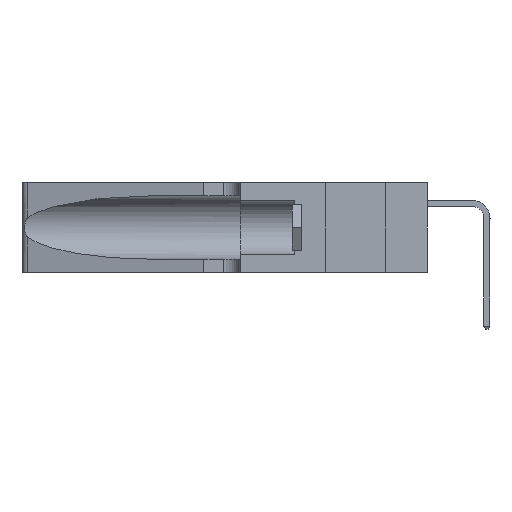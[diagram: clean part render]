
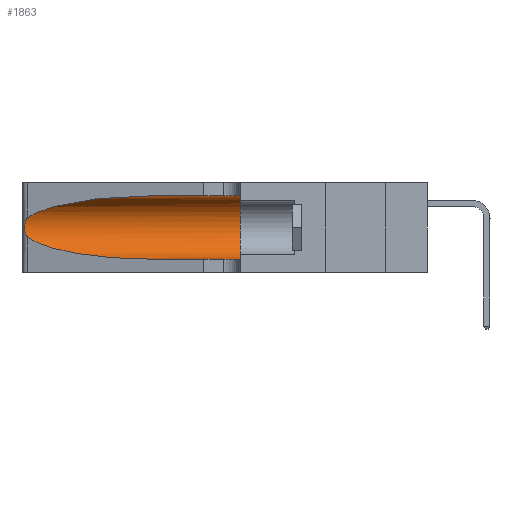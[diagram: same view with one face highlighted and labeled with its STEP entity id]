
A CAD part, left-side view. The second image highlights one B-rep face of the part: STEP entity #1863.
In plain terms, the highlighted cylindrical face has radius 3.308 mm (diameter 6.617 mm), a partial arc.
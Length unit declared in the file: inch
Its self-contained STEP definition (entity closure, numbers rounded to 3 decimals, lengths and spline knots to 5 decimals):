
#24 = DIRECTION ( 'NONE',  ( 0., 0., 1. ) ) ;
#83 = CARTESIAN_POINT ( 'NONE',  ( 0.1305, 0.35, 0.185 ) ) ;
#750 = DIRECTION ( 'NONE',  ( 0., -1., 0. ) ) ;
#790 = EDGE_CURVE ( 'NONE', #14074, #18296, #7745, .T. ) ;
#1110 = ORIENTED_EDGE ( 'NONE', *, *, #6047, .T. ) ;
#1334 = CARTESIAN_POINT ( 'NONE',  ( 0.25854, 1.2359, 0.20912 ) ) ;
#1863 = ADVANCED_FACE ( 'NONE', ( #5632 ), #17298, .F. ) ;
#2097 = LINE ( 'NONE', #19069, #5708 ) ;
#2897 = CARTESIAN_POINT ( 'NONE',  ( 0.26075, 1.23896, 0.19203 ) ) ;
#3001 = VECTOR ( 'NONE', #19380, 39.37008 ) ;
#3007 = CARTESIAN_POINT ( 'NONE',  ( 0.18966, 0.96281, 0.05475 ) ) ;
#3076 = B_SPLINE_CURVE_WITH_KNOTS ( 'NONE', 3,
 ( #5937, #13520, #19613, #10523, #1334, #12057, #2897, #13582, #4463, #15131, #6002, #16643, #7543, #18157 ),
 .UNSPECIFIED., .F., .F.,
 ( 4, 2, 2, 2, 2, 2, 4 ),
 ( 0., 0.00027, 0.00053, 0.00107, 0.0016, 0.00187, 0.00214 ),
 .UNSPECIFIED. ) ;
#3097 = VERTEX_POINT ( 'NONE', #10266 ) ;
#4463 = CARTESIAN_POINT ( 'NONE',  ( 0.26017, 1.23833, 0.17102 ) ) ;
#4508 = CARTESIAN_POINT ( 'NONE',  ( 0.25487, 1.22718, 0.14631 ) ) ;
#4941 = DIRECTION ( 'NONE',  ( 0., 1., 0. ) ) ;
#4996 = CARTESIAN_POINT ( 'NONE',  ( 0.18966, 0.96281, 0.31525 ) ) ;
#5586 = DIRECTION ( 'NONE',  ( 0., -1., 0. ) ) ;
#5632 = FACE_OUTER_BOUND ( 'NONE', #19132, .T. ) ;
#5708 = VECTOR ( 'NONE', #750, 39.37008 ) ;
#5758 = CARTESIAN_POINT ( 'NONE',  ( 0.1305, 1.61858, 0.31525 ) ) ;
#5937 = CARTESIAN_POINT ( 'NONE',  ( 0.25487, 1.22718, 0.22369 ) ) ;
#6002 = CARTESIAN_POINT ( 'NONE',  ( 0.25789, 1.23486, 0.15765 ) ) ;
#6047 = EDGE_CURVE ( 'NONE', #15755, #3097, #17273, .T. ) ;
#7324 = EDGE_CURVE ( 'NONE', #8057, #14074, #15196, .T. ) ;
#7543 = CARTESIAN_POINT ( 'NONE',  ( 0.25555, 1.22993, 0.14849 ) ) ;
#7589 = CARTESIAN_POINT ( 'NONE',  ( 0.2373, 1.15595, 0.08982 ) ) ;
#7745 = CIRCLE ( 'NONE', #16192, 0.13025 ) ;
#8057 = VERTEX_POINT ( 'NONE', #16905 ) ;
#8736 =( BOUNDED_CURVE ( )  B_SPLINE_CURVE ( 3, ( #9527, #4996, #18719, #9598 ),
 .UNSPECIFIED., .F., .F. ) 
 B_SPLINE_CURVE_WITH_KNOTS ( ( 4, 4 ),
 ( 1.5708, 2.84003 ),
 .UNSPECIFIED. ) 
 CURVE ( )  GEOMETRIC_REPRESENTATION_ITEM ( )  RATIONAL_B_SPLINE_CURVE ( ( 1., 0.87, 0.87, 1. ) ) 
 REPRESENTATION_ITEM ( '' )  );
#9527 = CARTESIAN_POINT ( 'NONE',  ( 0.1305, 0.72297, 0.31525 ) ) ;
#9598 = CARTESIAN_POINT ( 'NONE',  ( 0.25487, 1.22718, 0.22369 ) ) ;
#10266 = CARTESIAN_POINT ( 'NONE',  ( 0.1305, 0.72297, 0.05475 ) ) ;
#10523 = CARTESIAN_POINT ( 'NONE',  ( 0.25787, 1.23484, 0.2124 ) ) ;
#10882 = CARTESIAN_POINT ( 'NONE',  ( 0.25487, 1.22718, 0.14631 ) ) ;
#11413 = VERTEX_POINT ( 'NONE', #15230 ) ;
#11638 = CARTESIAN_POINT ( 'NONE',  ( 0.1305, 1.61858, 0.185 ) ) ;
#11886 = ORIENTED_EDGE ( 'NONE', *, *, #16187, .T. ) ;
#12057 = CARTESIAN_POINT ( 'NONE',  ( 0.26018, 1.23835, 0.19895 ) ) ;
#12684 = ORIENTED_EDGE ( 'NONE', *, *, #790, .F. ) ;
#12718 = ORIENTED_EDGE ( 'NONE', *, *, #7324, .F. ) ;
#13384 = EDGE_CURVE ( 'NONE', #3097, #18296, #2097, .T. ) ;
#13520 = CARTESIAN_POINT ( 'NONE',  ( 0.25555, 1.22994, 0.2215 ) ) ;
#13582 = CARTESIAN_POINT ( 'NONE',  ( 0.26075, 1.23896, 0.178 ) ) ;
#13698 = CARTESIAN_POINT ( 'NONE',  ( 0.1305, 0.72297, 0.05475 ) ) ;
#14074 = VERTEX_POINT ( 'NONE', #19047 ) ;
#15092 = CARTESIAN_POINT ( 'NONE',  ( 0.1305, 0.35, 0.05475 ) ) ;
#15131 = CARTESIAN_POINT ( 'NONE',  ( 0.25856, 1.23593, 0.16098 ) ) ;
#15196 = LINE ( 'NONE', #5758, #3001 ) ;
#15230 = CARTESIAN_POINT ( 'NONE',  ( 0.25487, 1.22718, 0.22369 ) ) ;
#15755 = VERTEX_POINT ( 'NONE', #10882 ) ;
#16087 = AXIS2_PLACEMENT_3D ( 'NONE', #11638, #5586, #19278 ) ;
#16187 = EDGE_CURVE ( 'NONE', #11413, #15755, #3076, .T. ) ;
#16192 = AXIS2_PLACEMENT_3D ( 'NONE', #83, #4941, #24 ) ;
#16643 = CARTESIAN_POINT ( 'NONE',  ( 0.25639, 1.23186, 0.15144 ) ) ;
#16905 = CARTESIAN_POINT ( 'NONE',  ( 0.1305, 0.72297, 0.31525 ) ) ;
#17273 =( BOUNDED_CURVE ( )  B_SPLINE_CURVE ( 3, ( #4508, #7589, #3007, #13698 ),
 .UNSPECIFIED., .F., .F. ) 
 B_SPLINE_CURVE_WITH_KNOTS ( ( 4, 4 ),
 ( 3.44316, 4.71239 ),
 .UNSPECIFIED. ) 
 CURVE ( )  GEOMETRIC_REPRESENTATION_ITEM ( )  RATIONAL_B_SPLINE_CURVE ( ( 1., 0.87, 0.87, 1. ) ) 
 REPRESENTATION_ITEM ( '' )  );
#17298 = CYLINDRICAL_SURFACE ( 'NONE', #16087, 0.13025 ) ;
#17435 = ORIENTED_EDGE ( 'NONE', *, *, #13384, .T. ) ;
#18157 = CARTESIAN_POINT ( 'NONE',  ( 0.25487, 1.22718, 0.14631 ) ) ;
#18296 = VERTEX_POINT ( 'NONE', #15092 ) ;
#18546 = EDGE_CURVE ( 'NONE', #8057, #11413, #8736, .T. ) ;
#18719 = CARTESIAN_POINT ( 'NONE',  ( 0.2373, 1.15595, 0.28018 ) ) ;
#19047 = CARTESIAN_POINT ( 'NONE',  ( 0.1305, 0.35, 0.31525 ) ) ;
#19069 = CARTESIAN_POINT ( 'NONE',  ( 0.1305, 1.61858, 0.05475 ) ) ;
#19132 = EDGE_LOOP ( 'NONE', ( #19314, #11886, #1110, #17435, #12684, #12718 ) ) ;
#19278 = DIRECTION ( 'NONE',  ( 0., 0., -1. ) ) ;
#19314 = ORIENTED_EDGE ( 'NONE', *, *, #18546, .T. ) ;
#19380 = DIRECTION ( 'NONE',  ( 0., -1., 0. ) ) ;
#19613 = CARTESIAN_POINT ( 'NONE',  ( 0.25639, 1.23184, 0.21858 ) ) ;
